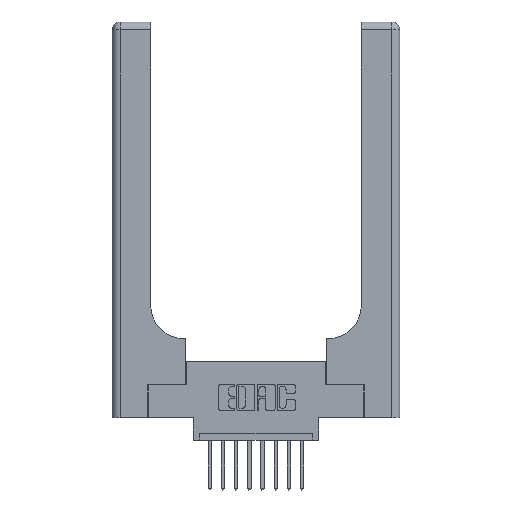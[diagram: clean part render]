
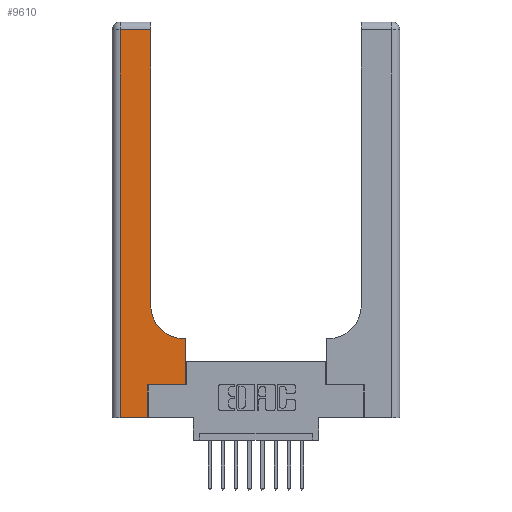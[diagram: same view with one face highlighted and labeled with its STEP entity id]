
A CAD part, top view. The second image highlights one B-rep face of the part: STEP entity #9610.
In plain terms, the highlighted planar face has unit normal (0, 0, 1).
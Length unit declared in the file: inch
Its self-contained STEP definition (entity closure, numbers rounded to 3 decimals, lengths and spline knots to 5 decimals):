
#116 = CARTESIAN_POINT ( 'NONE',  ( 0.269, 0., 0.37 ) ) ;
#291 = CARTESIAN_POINT ( 'NONE',  ( 0.269, 0., 0.37 ) ) ;
#438 = VERTEX_POINT ( 'NONE', #4180 ) ;
#2104 = ORIENTED_EDGE ( 'NONE', *, *, #2887, .T. ) ;
#2147 = LINE ( 'NONE', #116, #7563 ) ;
#2382 = VERTEX_POINT ( 'NONE', #10557 ) ;
#2697 = EDGE_CURVE ( 'NONE', #6321, #14930, #2147, .T. ) ;
#2887 = EDGE_CURVE ( 'NONE', #7666, #10484, #10027, .T. ) ;
#3217 = CARTESIAN_POINT ( 'NONE',  ( 0., 3., 0.37 ) ) ;
#3397 = CARTESIAN_POINT ( 'NONE',  ( 0.269, 0.25, 0.37 ) ) ;
#3486 = VERTEX_POINT ( 'NONE', #8113 ) ;
#3590 = DIRECTION ( 'NONE',  ( 0., 0., -1. ) ) ;
#3742 = LINE ( 'NONE', #4974, #13220 ) ;
#3849 = ORIENTED_EDGE ( 'NONE', *, *, #2697, .T. ) ;
#4180 = CARTESIAN_POINT ( 'NONE',  ( 0.5585, 0.25, 0.37 ) ) ;
#4223 = DIRECTION ( 'NONE',  ( 0., 1., 0. ) ) ;
#4258 = ORIENTED_EDGE ( 'NONE', *, *, #5117, .T. ) ;
#4376 = EDGE_CURVE ( 'NONE', #11549, #7666, #14845, .T. ) ;
#4880 = ORIENTED_EDGE ( 'NONE', *, *, #5219, .T. ) ;
#4933 = CARTESIAN_POINT ( 'NONE',  ( 0., 2.94, 0.37 ) ) ;
#4974 = CARTESIAN_POINT ( 'NONE',  ( 0.2915, 0.6, 0.37 ) ) ;
#5117 = EDGE_CURVE ( 'NONE', #14930, #438, #5775, .T. ) ;
#5219 = EDGE_CURVE ( 'NONE', #8388, #6321, #9406, .T. ) ;
#5616 = ORIENTED_EDGE ( 'NONE', *, *, #11187, .T. ) ;
#5775 = LINE ( 'NONE', #3397, #15415 ) ;
#6022 = CARTESIAN_POINT ( 'NONE',  ( 0.5415, 0.85, 0.37 ) ) ;
#6024 = DIRECTION ( 'NONE',  ( 1., 0., 0. ) ) ;
#6209 = CARTESIAN_POINT ( 'NONE',  ( 0.2915, 3., 0.37 ) ) ;
#6259 = CARTESIAN_POINT ( 'NONE',  ( 0.2915, 2.94, 0.37 ) ) ;
#6321 = VERTEX_POINT ( 'NONE', #291 ) ;
#6606 = CARTESIAN_POINT ( 'NONE',  ( 0.2915, 0.85, 0.37 ) ) ;
#6784 = VECTOR ( 'NONE', #13764, 39.37008 ) ;
#7550 = DIRECTION ( 'NONE',  ( 0., 1., 0. ) ) ;
#7563 = VECTOR ( 'NONE', #7550, 39.37008 ) ;
#7666 = VERTEX_POINT ( 'NONE', #6606 ) ;
#7954 = CARTESIAN_POINT ( 'NONE',  ( 0.269, 0.25, 0.37 ) ) ;
#8113 = CARTESIAN_POINT ( 'NONE',  ( 0.5585, 0.6, 0.37 ) ) ;
#8388 = VERTEX_POINT ( 'NONE', #12662 ) ;
#8643 = VECTOR ( 'NONE', #13942, 39.37008 ) ;
#8646 = EDGE_CURVE ( 'NONE', #10484, #2382, #15895, .T. ) ;
#8873 = EDGE_CURVE ( 'NONE', #438, #3486, #10489, .T. ) ;
#9326 = VECTOR ( 'NONE', #4223, 39.37008 ) ;
#9406 = LINE ( 'NONE', #11432, #8643 ) ;
#9430 = ORIENTED_EDGE ( 'NONE', *, *, #14202, .T. ) ;
#9610 = ADVANCED_FACE ( 'NONE', ( #15153 ), #10596, .F. ) ;
#9917 = DIRECTION ( 'NONE',  ( -1., 0., 0. ) ) ;
#10000 = EDGE_LOOP ( 'NONE', ( #2104, #14718, #5616, #4880, #3849, #4258, #12808, #9430, #10480 ) ) ;
#10008 = DIRECTION ( 'NONE',  ( -1., 0., 0. ) ) ;
#10027 = LINE ( 'NONE', #6209, #6784 ) ;
#10480 = ORIENTED_EDGE ( 'NONE', *, *, #4376, .T. ) ;
#10484 = VERTEX_POINT ( 'NONE', #6259 ) ;
#10489 = LINE ( 'NONE', #11105, #9326 ) ;
#10557 = CARTESIAN_POINT ( 'NONE',  ( 0.06, 2.94, 0.37 ) ) ;
#10596 = PLANE ( 'NONE',  #12112 ) ;
#11105 = CARTESIAN_POINT ( 'NONE',  ( 0.5585, 0.25, 0.37 ) ) ;
#11187 = EDGE_CURVE ( 'NONE', #2382, #8388, #15095, .T. ) ;
#11432 = CARTESIAN_POINT ( 'NONE',  ( 0., 0., 0.37 ) ) ;
#11549 = VERTEX_POINT ( 'NONE', #12642 ) ;
#11844 = CARTESIAN_POINT ( 'NONE',  ( 0.06, 3., 0.37 ) ) ;
#12112 = AXIS2_PLACEMENT_3D ( 'NONE', #3217, #3590, #13106 ) ;
#12642 = CARTESIAN_POINT ( 'NONE',  ( 0.5415, 0.6, 0.37 ) ) ;
#12662 = CARTESIAN_POINT ( 'NONE',  ( 0.06, 0., 0.37 ) ) ;
#12808 = ORIENTED_EDGE ( 'NONE', *, *, #8873, .T. ) ;
#13073 = DIRECTION ( 'NONE',  ( 0., -1., 0. ) ) ;
#13106 = DIRECTION ( 'NONE',  ( -1., 0., 0. ) ) ;
#13220 = VECTOR ( 'NONE', #10008, 39.37008 ) ;
#13435 = VECTOR ( 'NONE', #9917, 39.37008 ) ;
#13558 = DIRECTION ( 'NONE',  ( 0., 0., -1. ) ) ;
#13764 = DIRECTION ( 'NONE',  ( 0., 1., 0. ) ) ;
#13824 = AXIS2_PLACEMENT_3D ( 'NONE', #6022, #13558, #15885 ) ;
#13942 = DIRECTION ( 'NONE',  ( 1., 0., 0. ) ) ;
#14202 = EDGE_CURVE ( 'NONE', #3486, #11549, #3742, .T. ) ;
#14718 = ORIENTED_EDGE ( 'NONE', *, *, #8646, .T. ) ;
#14845 = CIRCLE ( 'NONE', #13824, 0.25 ) ;
#14930 = VERTEX_POINT ( 'NONE', #7954 ) ;
#15095 = LINE ( 'NONE', #11844, #15297 ) ;
#15153 = FACE_OUTER_BOUND ( 'NONE', #10000, .T. ) ;
#15297 = VECTOR ( 'NONE', #13073, 39.37008 ) ;
#15415 = VECTOR ( 'NONE', #6024, 39.37008 ) ;
#15885 = DIRECTION ( 'NONE',  ( 1., 0., 0. ) ) ;
#15895 = LINE ( 'NONE', #4933, #13435 ) ;
